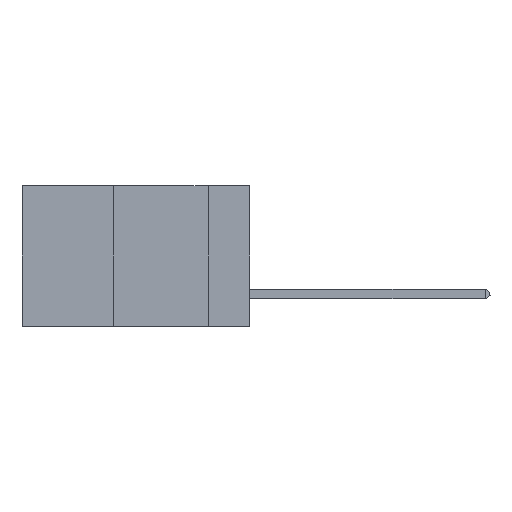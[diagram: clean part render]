
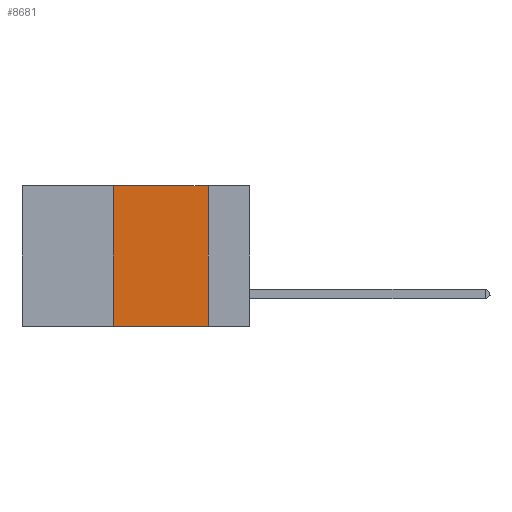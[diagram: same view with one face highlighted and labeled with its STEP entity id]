
A CAD part, left-side view. The second image highlights one B-rep face of the part: STEP entity #8681.
In plain terms, the highlighted planar face has unit normal (-1, 0, 0).
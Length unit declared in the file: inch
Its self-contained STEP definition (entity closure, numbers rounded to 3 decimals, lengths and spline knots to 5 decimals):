
#201 = VERTEX_POINT ( 'NONE', #10121 ) ;
#500 = EDGE_CURVE ( 'NONE', #11617, #10095, #13049, .T. ) ;
#676 = CARTESIAN_POINT ( 'NONE',  ( 0., 0.6, 0. ) ) ;
#923 = DIRECTION ( 'NONE',  ( 1., 0., 0. ) ) ;
#2166 = CARTESIAN_POINT ( 'NONE',  ( 0., 0.36, 0. ) ) ;
#2188 = LINE ( 'NONE', #2166, #16588 ) ;
#2203 = DIRECTION ( 'NONE',  ( 0., 0., -1. ) ) ;
#2587 = ORIENTED_EDGE ( 'NONE', *, *, #10727, .F. ) ;
#3075 = CARTESIAN_POINT ( 'NONE',  ( 0., 0.11, -0.37 ) ) ;
#3490 = DIRECTION ( 'NONE',  ( 0., -1., 0. ) ) ;
#3520 = ORIENTED_EDGE ( 'NONE', *, *, #4351, .F. ) ;
#4351 = EDGE_CURVE ( 'NONE', #11617, #201, #2188, .T. ) ;
#4764 = AXIS2_PLACEMENT_3D ( 'NONE', #676, #923, #2203 ) ;
#4780 = VERTEX_POINT ( 'NONE', #14722 ) ;
#5015 = EDGE_CURVE ( 'NONE', #201, #4780, #10047, .T. ) ;
#5756 = CARTESIAN_POINT ( 'NONE',  ( 0., 0.11, 0. ) ) ;
#7445 = CARTESIAN_POINT ( 'NONE',  ( 0., 0.6, -0.37 ) ) ;
#8302 = DIRECTION ( 'NONE',  ( 0., 0., -1. ) ) ;
#8517 = CARTESIAN_POINT ( 'NONE',  ( 0., 0.6, 0. ) ) ;
#8681 = ADVANCED_FACE ( 'NONE', ( #9177 ), #14840, .F. ) ;
#9100 = VECTOR ( 'NONE', #3490, 39.37008 ) ;
#9177 = FACE_OUTER_BOUND ( 'NONE', #17956, .T. ) ;
#10047 = LINE ( 'NONE', #8517, #17912 ) ;
#10095 = VERTEX_POINT ( 'NONE', #3075 ) ;
#10121 = CARTESIAN_POINT ( 'NONE',  ( 0., 0.36, 0. ) ) ;
#10715 = DIRECTION ( 'NONE',  ( 0., 0., 1. ) ) ;
#10727 = EDGE_CURVE ( 'NONE', #4780, #10095, #11097, .T. ) ;
#11097 = LINE ( 'NONE', #5756, #15227 ) ;
#11118 = CARTESIAN_POINT ( 'NONE',  ( 0., 0.36, -0.37 ) ) ;
#11617 = VERTEX_POINT ( 'NONE', #11118 ) ;
#12884 = DIRECTION ( 'NONE',  ( 0., -1., 0. ) ) ;
#12943 = ORIENTED_EDGE ( 'NONE', *, *, #500, .T. ) ;
#13049 = LINE ( 'NONE', #7445, #9100 ) ;
#14722 = CARTESIAN_POINT ( 'NONE',  ( 0., 0.11, 0. ) ) ;
#14840 = PLANE ( 'NONE',  #4764 ) ;
#15227 = VECTOR ( 'NONE', #8302, 39.37008 ) ;
#16143 = ORIENTED_EDGE ( 'NONE', *, *, #5015, .F. ) ;
#16588 = VECTOR ( 'NONE', #10715, 39.37008 ) ;
#17912 = VECTOR ( 'NONE', #12884, 39.37008 ) ;
#17956 = EDGE_LOOP ( 'NONE', ( #2587, #16143, #3520, #12943 ) ) ;
